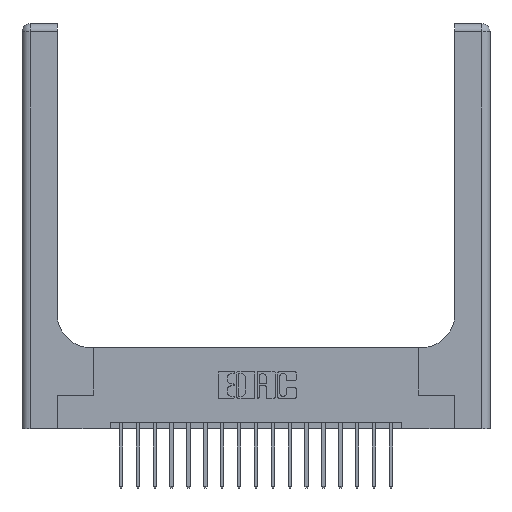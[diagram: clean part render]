
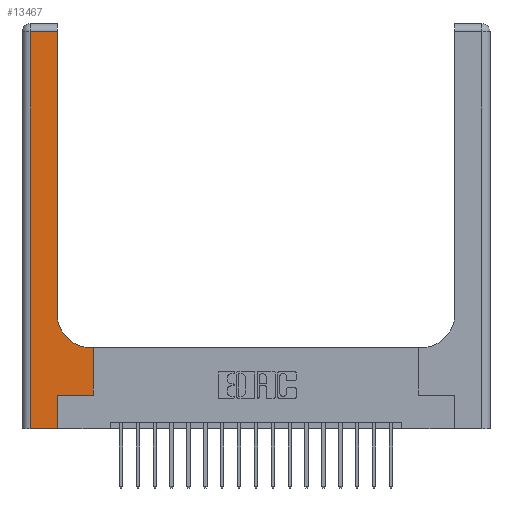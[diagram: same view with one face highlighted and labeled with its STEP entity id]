
A CAD part, top view. The second image highlights one B-rep face of the part: STEP entity #13467.
In plain terms, the highlighted planar face has unit normal (0, 0, 1).
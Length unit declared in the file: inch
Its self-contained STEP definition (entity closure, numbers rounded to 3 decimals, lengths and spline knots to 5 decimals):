
#2 = VECTOR ( 'NONE', #18839, 39.37008 ) ;
#118 = CARTESIAN_POINT ( 'NONE',  ( 0.26, 0.6, 0.37 ) ) ;
#233 = DIRECTION ( 'NONE',  ( -1., 0., 0. ) ) ;
#337 = EDGE_LOOP ( 'NONE', ( #569, #3070, #15210, #8967, #3059, #15333, #19340, #4762, #18556 ) ) ;
#453 = CARTESIAN_POINT ( 'NONE',  ( 0., 0., 0.37 ) ) ;
#569 = ORIENTED_EDGE ( 'NONE', *, *, #4144, .T. ) ;
#970 = VECTOR ( 'NONE', #16378, 39.37008 ) ;
#1238 = CARTESIAN_POINT ( 'NONE',  ( 0.06, 3., 0.37 ) ) ;
#1445 = DIRECTION ( 'NONE',  ( 0., -1., 0. ) ) ;
#2057 = EDGE_CURVE ( 'NONE', #14817, #17760, #10553, .T. ) ;
#2112 = VERTEX_POINT ( 'NONE', #10281 ) ;
#2186 = LINE ( 'NONE', #2923, #970 ) ;
#2220 = CARTESIAN_POINT ( 'NONE',  ( 0., 2.94, 0.37 ) ) ;
#2923 = CARTESIAN_POINT ( 'NONE',  ( 0.26, 3., 0.37 ) ) ;
#2925 = EDGE_CURVE ( 'NONE', #2112, #13675, #7484, .T. ) ;
#3059 = ORIENTED_EDGE ( 'NONE', *, *, #13945, .T. ) ;
#3070 = ORIENTED_EDGE ( 'NONE', *, *, #15290, .T. ) ;
#3154 = LINE ( 'NONE', #118, #14059 ) ;
#3988 = VERTEX_POINT ( 'NONE', #18582 ) ;
#4019 = CARTESIAN_POINT ( 'NONE',  ( 0.26, 0.85, 0.37 ) ) ;
#4144 = EDGE_CURVE ( 'NONE', #13675, #3988, #2186, .T. ) ;
#4222 = DIRECTION ( 'NONE',  ( 0., 1., 0. ) ) ;
#4284 = CARTESIAN_POINT ( 'NONE',  ( 0.528, 0.6, 0.37 ) ) ;
#4335 = VECTOR ( 'NONE', #9611, 39.37008 ) ;
#4395 = EDGE_CURVE ( 'NONE', #18141, #10226, #14247, .T. ) ;
#4762 = ORIENTED_EDGE ( 'NONE', *, *, #16640, .T. ) ;
#5114 = EDGE_CURVE ( 'NONE', #16207, #14817, #10424, .T. ) ;
#5248 = DIRECTION ( 'NONE',  ( 0., 1., 0. ) ) ;
#5604 = VECTOR ( 'NONE', #1445, 39.37008 ) ;
#5667 = DIRECTION ( 'NONE',  ( -1., 0., 0. ) ) ;
#5830 = CARTESIAN_POINT ( 'NONE',  ( 0.528, 0.25, 0.37 ) ) ;
#7181 = DIRECTION ( 'NONE',  ( 0., 0., -1. ) ) ;
#7253 = DIRECTION ( 'NONE',  ( -1., 0., 0. ) ) ;
#7323 = VERTEX_POINT ( 'NONE', #15490 ) ;
#7484 = CIRCLE ( 'NONE', #9630, 0.25 ) ;
#7517 = AXIS2_PLACEMENT_3D ( 'NONE', #12426, #9331, #233 ) ;
#7579 = VECTOR ( 'NONE', #5248, 39.37008 ) ;
#7965 = PLANE ( 'NONE',  #7517 ) ;
#8422 = CARTESIAN_POINT ( 'NONE',  ( 0.265, 0., 0.37 ) ) ;
#8434 = FACE_OUTER_BOUND ( 'NONE', #337, .T. ) ;
#8456 = VECTOR ( 'NONE', #4222, 39.37008 ) ;
#8967 = ORIENTED_EDGE ( 'NONE', *, *, #4395, .T. ) ;
#9331 = DIRECTION ( 'NONE',  ( 0., 0., -1. ) ) ;
#9611 = DIRECTION ( 'NONE',  ( 1., 0., 0. ) ) ;
#9621 = LINE ( 'NONE', #1238, #5604 ) ;
#9630 = AXIS2_PLACEMENT_3D ( 'NONE', #14407, #7181, #17603 ) ;
#9672 = CARTESIAN_POINT ( 'NONE',  ( 0.265, 0., 0.37 ) ) ;
#10085 = VECTOR ( 'NONE', #5667, 39.37008 ) ;
#10226 = VERTEX_POINT ( 'NONE', #8422 ) ;
#10281 = CARTESIAN_POINT ( 'NONE',  ( 0.51, 0.6, 0.37 ) ) ;
#10424 = LINE ( 'NONE', #12641, #2 ) ;
#10553 = LINE ( 'NONE', #19121, #8456 ) ;
#10844 = LINE ( 'NONE', #9672, #7579 ) ;
#12426 = CARTESIAN_POINT ( 'NONE',  ( 0., 3., 0.37 ) ) ;
#12641 = CARTESIAN_POINT ( 'NONE',  ( 0.265, 0.25, 0.37 ) ) ;
#13467 = ADVANCED_FACE ( 'NONE', ( #8434 ), #7965, .F. ) ;
#13675 = VERTEX_POINT ( 'NONE', #4019 ) ;
#13945 = EDGE_CURVE ( 'NONE', #10226, #16207, #10844, .T. ) ;
#14059 = VECTOR ( 'NONE', #7253, 39.37008 ) ;
#14247 = LINE ( 'NONE', #453, #4335 ) ;
#14407 = CARTESIAN_POINT ( 'NONE',  ( 0.51, 0.85, 0.37 ) ) ;
#14817 = VERTEX_POINT ( 'NONE', #5830 ) ;
#15210 = ORIENTED_EDGE ( 'NONE', *, *, #15524, .T. ) ;
#15290 = EDGE_CURVE ( 'NONE', #3988, #7323, #19120, .T. ) ;
#15333 = ORIENTED_EDGE ( 'NONE', *, *, #5114, .T. ) ;
#15490 = CARTESIAN_POINT ( 'NONE',  ( 0.06, 2.94, 0.37 ) ) ;
#15524 = EDGE_CURVE ( 'NONE', #7323, #18141, #9621, .T. ) ;
#16207 = VERTEX_POINT ( 'NONE', #16421 ) ;
#16378 = DIRECTION ( 'NONE',  ( 0., 1., 0. ) ) ;
#16421 = CARTESIAN_POINT ( 'NONE',  ( 0.265, 0.25, 0.37 ) ) ;
#16640 = EDGE_CURVE ( 'NONE', #17760, #2112, #3154, .T. ) ;
#17176 = CARTESIAN_POINT ( 'NONE',  ( 0.06, 0., 0.37 ) ) ;
#17603 = DIRECTION ( 'NONE',  ( 1., 0., 0. ) ) ;
#17760 = VERTEX_POINT ( 'NONE', #4284 ) ;
#18141 = VERTEX_POINT ( 'NONE', #17176 ) ;
#18556 = ORIENTED_EDGE ( 'NONE', *, *, #2925, .T. ) ;
#18582 = CARTESIAN_POINT ( 'NONE',  ( 0.26, 2.94, 0.37 ) ) ;
#18839 = DIRECTION ( 'NONE',  ( 1., 0., 0. ) ) ;
#19120 = LINE ( 'NONE', #2220, #10085 ) ;
#19121 = CARTESIAN_POINT ( 'NONE',  ( 0.528, 0.25, 0.37 ) ) ;
#19340 = ORIENTED_EDGE ( 'NONE', *, *, #2057, .T. ) ;
